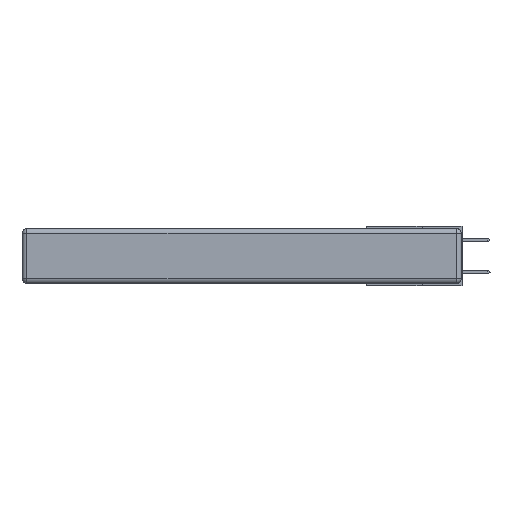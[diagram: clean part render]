
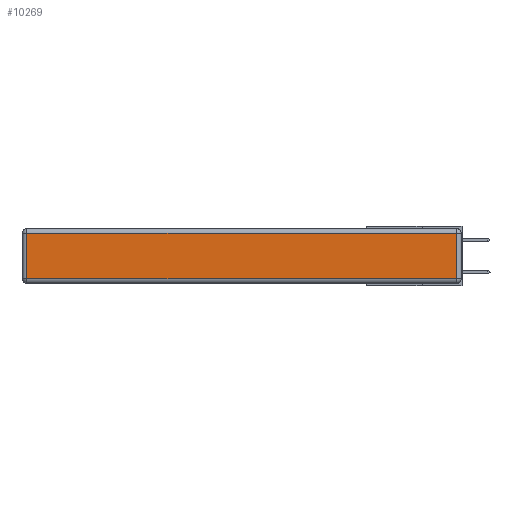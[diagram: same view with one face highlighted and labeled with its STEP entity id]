
A CAD part, left-side view. The second image highlights one B-rep face of the part: STEP entity #10269.
In plain terms, the highlighted planar face has unit normal (-1, 0, 0).
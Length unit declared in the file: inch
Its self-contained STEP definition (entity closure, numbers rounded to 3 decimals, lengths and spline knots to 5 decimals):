
#1147 = VERTEX_POINT ( 'NONE', #1788 ) ;
#1788 = CARTESIAN_POINT ( 'NONE',  ( 0., 0.03, -0.03 ) ) ;
#3340 = DIRECTION ( 'NONE',  ( 0., 0., -1. ) ) ;
#3642 = DIRECTION ( 'NONE',  ( 0., 0., 1. ) ) ;
#4223 = CARTESIAN_POINT ( 'NONE',  ( 0., 0., -0.343 ) ) ;
#4986 = EDGE_LOOP ( 'NONE', ( #18872, #7852, #7354, #6531 ) ) ;
#5099 = CARTESIAN_POINT ( 'NONE',  ( 0., 0., -0.313 ) ) ;
#6531 = ORIENTED_EDGE ( 'NONE', *, *, #9533, .T. ) ;
#7354 = ORIENTED_EDGE ( 'NONE', *, *, #24008, .T. ) ;
#7852 = ORIENTED_EDGE ( 'NONE', *, *, #19958, .T. ) ;
#7923 = DIRECTION ( 'NONE',  ( 0., 0., 1. ) ) ;
#8549 = LINE ( 'NONE', #5099, #8856 ) ;
#8856 = VECTOR ( 'NONE', #16240, 39.37008 ) ;
#8868 = CARTESIAN_POINT ( 'NONE',  ( 0., 0.03, -0.313 ) ) ;
#8909 = CARTESIAN_POINT ( 'NONE',  ( 0., 2.72, -0.343 ) ) ;
#9533 = EDGE_CURVE ( 'NONE', #13079, #22881, #14213, .T. ) ;
#9746 = FACE_OUTER_BOUND ( 'NONE', #4986, .T. ) ;
#10264 = LINE ( 'NONE', #14901, #11460 ) ;
#10269 = ADVANCED_FACE ( 'NONE', ( #9746 ), #11936, .T. ) ;
#10362 = AXIS2_PLACEMENT_3D ( 'NONE', #4223, #17339, #7923 ) ;
#10511 = EDGE_CURVE ( 'NONE', #22881, #22445, #8549, .T. ) ;
#11460 = VECTOR ( 'NONE', #3642, 39.37008 ) ;
#11602 = CARTESIAN_POINT ( 'NONE',  ( 0., 2.72, -0.313 ) ) ;
#11936 = PLANE ( 'NONE',  #10362 ) ;
#13079 = VERTEX_POINT ( 'NONE', #21263 ) ;
#13112 = DIRECTION ( 'NONE',  ( 0., 1., 0. ) ) ;
#14213 = LINE ( 'NONE', #8909, #18087 ) ;
#14901 = CARTESIAN_POINT ( 'NONE',  ( 0., 0.03, -0.343 ) ) ;
#15140 = LINE ( 'NONE', #16688, #16620 ) ;
#16240 = DIRECTION ( 'NONE',  ( 0., -1., 0. ) ) ;
#16620 = VECTOR ( 'NONE', #13112, 39.37008 ) ;
#16688 = CARTESIAN_POINT ( 'NONE',  ( 0., 2.75, -0.03 ) ) ;
#17339 = DIRECTION ( 'NONE',  ( -1., 0., 0. ) ) ;
#18087 = VECTOR ( 'NONE', #3340, 39.37008 ) ;
#18872 = ORIENTED_EDGE ( 'NONE', *, *, #10511, .T. ) ;
#19958 = EDGE_CURVE ( 'NONE', #22445, #1147, #10264, .T. ) ;
#21263 = CARTESIAN_POINT ( 'NONE',  ( 0., 2.72, -0.03 ) ) ;
#22445 = VERTEX_POINT ( 'NONE', #8868 ) ;
#22881 = VERTEX_POINT ( 'NONE', #11602 ) ;
#24008 = EDGE_CURVE ( 'NONE', #1147, #13079, #15140, .T. ) ;
